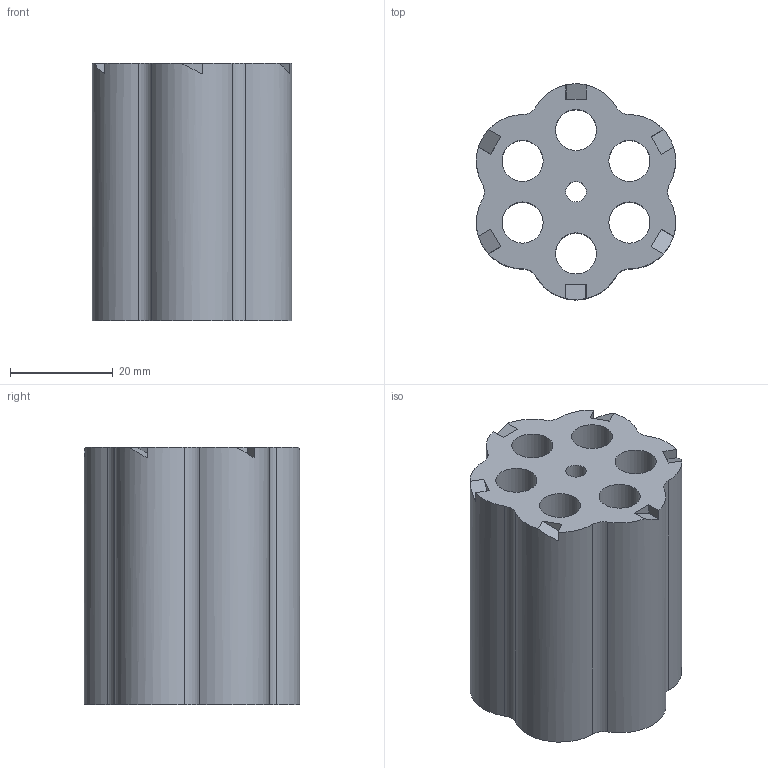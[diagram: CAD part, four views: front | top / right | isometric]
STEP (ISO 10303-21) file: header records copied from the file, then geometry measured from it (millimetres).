
FILE_DESCRIPTION((''),'2;1');
FILE_NAME('barrel.stp','2013-08-15T20:09:26',('mrfr'),(''),'Autodesk Inventor 2013','Autodesk Inventor 2013','');
FILE_SCHEMA(('AUTOMOTIVE_DESIGN { 1 0 10303 214 1 1 1 1 }'));
Length unit declared in the file: millimetre
Products named in the file (1): barrel
Bounding box: 38.78 x 42 x 50 mm (x, y, z)
Volume: 45477.4 mm3; surface area: 16699.3 mm2
Topology: 1 solids, 1 shells, 47 faces, 133 edges, 89 vertices
Faces by surface type: plane 27, cylinder 20
Full cylindrical faces by diameter (mm): 4 x1, 8 x7
Entity records: 1558 total; most frequent: DIRECTION 278, CARTESIAN_POINT 260, ORIENTED_EDGE 248, EDGE_CURVE 124, AXIS2_PLACEMENT_3D 106, VERTEX_POINT 88, EDGE_LOOP 70, VECTOR 66
